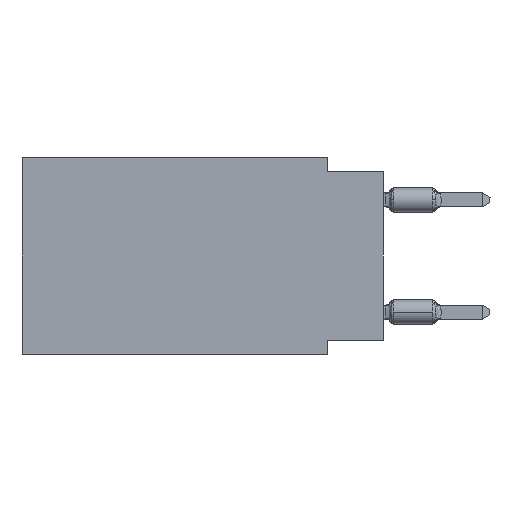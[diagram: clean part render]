
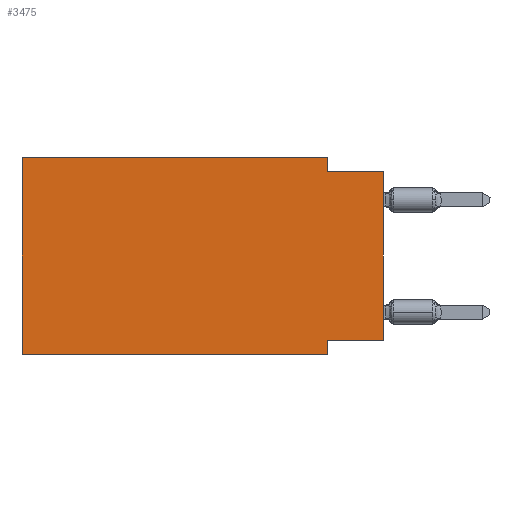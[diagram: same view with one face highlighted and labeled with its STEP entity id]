
A CAD part, left-side view. The second image highlights one B-rep face of the part: STEP entity #3475.
In plain terms, the highlighted planar face has unit normal (-1, 0, 0).
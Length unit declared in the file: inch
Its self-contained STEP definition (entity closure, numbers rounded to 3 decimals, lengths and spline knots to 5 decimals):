
#37 = ORIENTED_EDGE ( 'NONE', *, *, #18921, .F. ) ;
#500 = VERTEX_POINT ( 'NONE', #4083 ) ;
#1979 = CARTESIAN_POINT ( 'NONE',  ( 0., 0., -0.325 ) ) ;
#3475 = ADVANCED_FACE ( 'NONE', ( #31416 ), #6437, .F. ) ;
#4083 = CARTESIAN_POINT ( 'NONE',  ( 0., 0.1, -0.025 ) ) ;
#5019 = EDGE_CURVE ( 'NONE', #44936, #11888, #28125, .T. ) ;
#6437 = PLANE ( 'NONE',  #10878 ) ;
#7247 = LINE ( 'NONE', #48352, #45219 ) ;
#8087 = LINE ( 'NONE', #16635, #22437 ) ;
#8418 = CARTESIAN_POINT ( 'NONE',  ( 0., 0.645, 0. ) ) ;
#8577 = DIRECTION ( 'NONE',  ( 0., -1., 0. ) ) ;
#9298 = EDGE_CURVE ( 'NONE', #41051, #23541, #40632, .T. ) ;
#9646 = EDGE_CURVE ( 'NONE', #41078, #500, #25038, .T. ) ;
#9889 = DIRECTION ( 'NONE',  ( 1., 0., 0. ) ) ;
#10878 = AXIS2_PLACEMENT_3D ( 'NONE', #25037, #9889, #36292 ) ;
#11888 = VERTEX_POINT ( 'NONE', #15190 ) ;
#13312 = ORIENTED_EDGE ( 'NONE', *, *, #38519, .F. ) ;
#13476 = DIRECTION ( 'NONE',  ( 0., 0., 1. ) ) ;
#15190 = CARTESIAN_POINT ( 'NONE',  ( 0., 0., -0.025 ) ) ;
#15608 = CARTESIAN_POINT ( 'NONE',  ( 0., 0.645, -0.35 ) ) ;
#16635 = CARTESIAN_POINT ( 'NONE',  ( 0., 0., -0.025 ) ) ;
#17574 = DIRECTION ( 'NONE',  ( 0., -1., 0. ) ) ;
#18732 = ORIENTED_EDGE ( 'NONE', *, *, #9298, .F. ) ;
#18921 = EDGE_CURVE ( 'NONE', #500, #11888, #8087, .T. ) ;
#19603 = ORIENTED_EDGE ( 'NONE', *, *, #21950, .F. ) ;
#21554 = EDGE_CURVE ( 'NONE', #33955, #23541, #38095, .T. ) ;
#21950 = EDGE_CURVE ( 'NONE', #44936, #41051, #32319, .T. ) ;
#22325 = VERTEX_POINT ( 'NONE', #27629 ) ;
#22437 = VECTOR ( 'NONE', #8577, 39.37008 ) ;
#22720 = ORIENTED_EDGE ( 'NONE', *, *, #47836, .F. ) ;
#23416 = DIRECTION ( 'NONE',  ( 0., -1., 0. ) ) ;
#23541 = VERTEX_POINT ( 'NONE', #28454 ) ;
#25037 = CARTESIAN_POINT ( 'NONE',  ( 0., 0.645, 0. ) ) ;
#25038 = LINE ( 'NONE', #32629, #40968 ) ;
#26291 = CARTESIAN_POINT ( 'NONE',  ( 0., 0.1, -0.325 ) ) ;
#26686 = CARTESIAN_POINT ( 'NONE',  ( 0., 0.1, -0.35 ) ) ;
#27629 = CARTESIAN_POINT ( 'NONE',  ( 0., 0.645, 0. ) ) ;
#28125 = LINE ( 'NONE', #28619, #34494 ) ;
#28454 = CARTESIAN_POINT ( 'NONE',  ( 0., 0.1, -0.35 ) ) ;
#28619 = CARTESIAN_POINT ( 'NONE',  ( 0., 0., 0. ) ) ;
#28637 = DIRECTION ( 'NONE',  ( 0., 1., 0. ) ) ;
#28649 = EDGE_LOOP ( 'NONE', ( #35794, #37, #29973, #13312, #22720, #48251, #18732, #19603 ) ) ;
#29088 = CARTESIAN_POINT ( 'NONE',  ( 0., 0.645, -0.35 ) ) ;
#29601 = DIRECTION ( 'NONE',  ( 0., 0., -1. ) ) ;
#29973 = ORIENTED_EDGE ( 'NONE', *, *, #9646, .F. ) ;
#30483 = VECTOR ( 'NONE', #28637, 39.37008 ) ;
#31416 = FACE_OUTER_BOUND ( 'NONE', #28649, .T. ) ;
#32319 = LINE ( 'NONE', #1979, #30483 ) ;
#32629 = CARTESIAN_POINT ( 'NONE',  ( 0., 0.1, 0. ) ) ;
#33955 = VERTEX_POINT ( 'NONE', #29088 ) ;
#34113 = CARTESIAN_POINT ( 'NONE',  ( 0., 0.1, 0. ) ) ;
#34494 = VECTOR ( 'NONE', #13476, 39.37008 ) ;
#35794 = ORIENTED_EDGE ( 'NONE', *, *, #5019, .T. ) ;
#36292 = DIRECTION ( 'NONE',  ( 0., 0., -1. ) ) ;
#36457 = CARTESIAN_POINT ( 'NONE',  ( 0., 0., -0.325 ) ) ;
#36684 = VECTOR ( 'NONE', #23416, 39.37008 ) ;
#38095 = LINE ( 'NONE', #15608, #36684 ) ;
#38519 = EDGE_CURVE ( 'NONE', #22325, #41078, #7247, .T. ) ;
#40632 = LINE ( 'NONE', #26686, #42530 ) ;
#40968 = VECTOR ( 'NONE', #47547, 39.37008 ) ;
#41051 = VERTEX_POINT ( 'NONE', #26291 ) ;
#41078 = VERTEX_POINT ( 'NONE', #34113 ) ;
#41587 = VECTOR ( 'NONE', #44857, 39.37008 ) ;
#42158 = LINE ( 'NONE', #8418, #41587 ) ;
#42530 = VECTOR ( 'NONE', #29601, 39.37008 ) ;
#44857 = DIRECTION ( 'NONE',  ( 0., 0., 1. ) ) ;
#44936 = VERTEX_POINT ( 'NONE', #36457 ) ;
#45219 = VECTOR ( 'NONE', #17574, 39.37008 ) ;
#47547 = DIRECTION ( 'NONE',  ( 0., 0., -1. ) ) ;
#47836 = EDGE_CURVE ( 'NONE', #33955, #22325, #42158, .T. ) ;
#48251 = ORIENTED_EDGE ( 'NONE', *, *, #21554, .T. ) ;
#48352 = CARTESIAN_POINT ( 'NONE',  ( 0., 0.645, 0. ) ) ;
